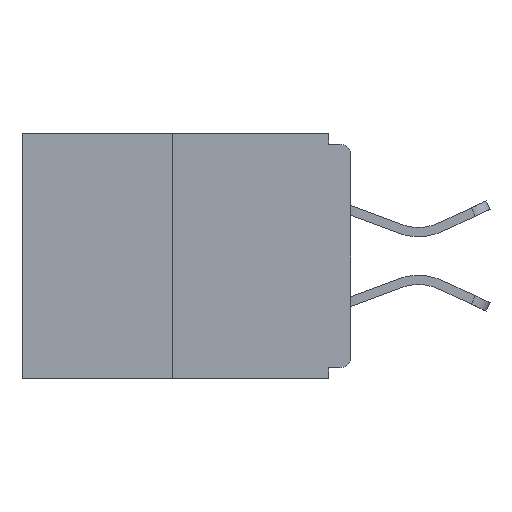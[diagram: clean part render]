
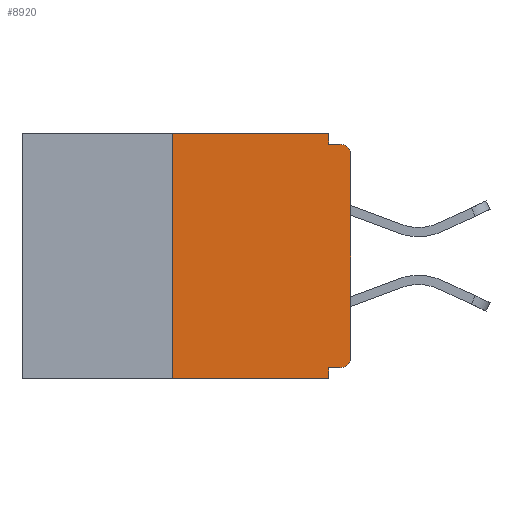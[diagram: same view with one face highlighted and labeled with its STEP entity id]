
A CAD part, left-side view. The second image highlights one B-rep face of the part: STEP entity #8920.
In plain terms, the highlighted planar face has unit normal (-1, 0, 0).
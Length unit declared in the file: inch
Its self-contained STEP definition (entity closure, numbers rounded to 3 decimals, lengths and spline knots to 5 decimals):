
#561 = LINE ( 'NONE', #5467, #5414 ) ;
#595 = VECTOR ( 'NONE', #7251, 39.37008 ) ;
#727 = VERTEX_POINT ( 'NONE', #7992 ) ;
#824 = DIRECTION ( 'NONE',  ( 0., 0., -1. ) ) ;
#912 = VECTOR ( 'NONE', #824, 39.37008 ) ;
#916 = VERTEX_POINT ( 'NONE', #6144 ) ;
#1328 = DIRECTION ( 'NONE',  ( 0., 0., -1. ) ) ;
#1389 = AXIS2_PLACEMENT_3D ( 'NONE', #11991, #3288, #1328 ) ;
#1427 = VECTOR ( 'NONE', #3119, 39.37008 ) ;
#1448 = EDGE_LOOP ( 'NONE', ( #5956, #11105, #6914, #5682, #10189, #10742, #6985, #7976, #5440, #7328 ) ) ;
#1656 = EDGE_CURVE ( 'NONE', #5691, #10394, #11904, .T. ) ;
#1929 = CARTESIAN_POINT ( 'NONE',  ( 0., 0.015, -0.328 ) ) ;
#1949 = PLANE ( 'NONE',  #9711 ) ;
#2046 = FACE_OUTER_BOUND ( 'NONE', #1448, .T. ) ;
#2208 = VERTEX_POINT ( 'NONE', #10287 ) ;
#2291 = CARTESIAN_POINT ( 'NONE',  ( 0., 0., -0.03 ) ) ;
#2743 = CARTESIAN_POINT ( 'NONE',  ( 0., 0.031, 0. ) ) ;
#2788 = DIRECTION ( 'NONE',  ( 0., -1., 0. ) ) ;
#2835 = EDGE_CURVE ( 'NONE', #2208, #5691, #561, .T. ) ;
#3022 = DIRECTION ( 'NONE',  ( 1., 0., 0. ) ) ;
#3119 = DIRECTION ( 'NONE',  ( 0., -1., 0. ) ) ;
#3155 = VERTEX_POINT ( 'NONE', #2291 ) ;
#3254 = CARTESIAN_POINT ( 'NONE',  ( 0., 0.015, -0.015 ) ) ;
#3288 = DIRECTION ( 'NONE',  ( -1., 0., 0. ) ) ;
#3800 = CIRCLE ( 'NONE', #1389, 0.015 ) ;
#3855 = LINE ( 'NONE', #7101, #1427 ) ;
#3993 = DIRECTION ( 'NONE',  ( 0., 0., -1. ) ) ;
#4251 = CARTESIAN_POINT ( 'NONE',  ( 0., 0.031, 0. ) ) ;
#4756 = CARTESIAN_POINT ( 'NONE',  ( 0., 0., -0.328 ) ) ;
#4783 = EDGE_CURVE ( 'NONE', #3155, #12148, #7223, .T. ) ;
#5377 = DIRECTION ( 'NONE',  ( 0., -1., 0. ) ) ;
#5414 = VECTOR ( 'NONE', #11249, 39.37008 ) ;
#5440 = ORIENTED_EDGE ( 'NONE', *, *, #6871, .F. ) ;
#5467 = CARTESIAN_POINT ( 'NONE',  ( 0., 0.25, 0. ) ) ;
#5682 = ORIENTED_EDGE ( 'NONE', *, *, #10095, .F. ) ;
#5691 = VERTEX_POINT ( 'NONE', #10473 ) ;
#5806 = LINE ( 'NONE', #11042, #9380 ) ;
#5827 = EDGE_CURVE ( 'NONE', #10600, #12441, #3800, .T. ) ;
#5956 = ORIENTED_EDGE ( 'NONE', *, *, #1656, .F. ) ;
#6078 = LINE ( 'NONE', #2743, #912 ) ;
#6144 = CARTESIAN_POINT ( 'NONE',  ( 0., 0.031, -0.328 ) ) ;
#6581 = EDGE_CURVE ( 'NONE', #12441, #3155, #10989, .T. ) ;
#6602 = DIRECTION ( 'NONE',  ( 0., 1., 0. ) ) ;
#6702 = CARTESIAN_POINT ( 'NONE',  ( 0., 0.46, 0. ) ) ;
#6709 = CARTESIAN_POINT ( 'NONE',  ( 0., 0., -0.015 ) ) ;
#6871 = EDGE_CURVE ( 'NONE', #12195, #12148, #9323, .T. ) ;
#6914 = ORIENTED_EDGE ( 'NONE', *, *, #11793, .T. ) ;
#6965 = EDGE_CURVE ( 'NONE', #10600, #916, #10816, .T. ) ;
#6985 = ORIENTED_EDGE ( 'NONE', *, *, #6581, .T. ) ;
#7101 = CARTESIAN_POINT ( 'NONE',  ( 0., 0.46, -0.343 ) ) ;
#7223 = CIRCLE ( 'NONE', #8395, 0.015 ) ;
#7251 = DIRECTION ( 'NONE',  ( 0., 0., 1. ) ) ;
#7328 = ORIENTED_EDGE ( 'NONE', *, *, #11694, .F. ) ;
#7502 = CARTESIAN_POINT ( 'NONE',  ( 0., 0.46, 0. ) ) ;
#7670 = DIRECTION ( 'NONE',  ( 0., 0., -1. ) ) ;
#7976 = ORIENTED_EDGE ( 'NONE', *, *, #4783, .T. ) ;
#7992 = CARTESIAN_POINT ( 'NONE',  ( 0., 0.031, -0.343 ) ) ;
#8254 = CARTESIAN_POINT ( 'NONE',  ( 0., 0.031, -0.015 ) ) ;
#8395 = AXIS2_PLACEMENT_3D ( 'NONE', #9520, #12278, #7670 ) ;
#8530 = CARTESIAN_POINT ( 'NONE',  ( 0., 0., -0.313 ) ) ;
#8920 = ADVANCED_FACE ( 'NONE', ( #2046 ), #1949, .F. ) ;
#9323 = LINE ( 'NONE', #6709, #9467 ) ;
#9380 = VECTOR ( 'NONE', #10999, 39.37008 ) ;
#9467 = VECTOR ( 'NONE', #2788, 39.37008 ) ;
#9520 = CARTESIAN_POINT ( 'NONE',  ( 0., 0.015, -0.03 ) ) ;
#9711 = AXIS2_PLACEMENT_3D ( 'NONE', #6702, #3022, #3993 ) ;
#10095 = EDGE_CURVE ( 'NONE', #916, #727, #5806, .T. ) ;
#10189 = ORIENTED_EDGE ( 'NONE', *, *, #6965, .F. ) ;
#10287 = CARTESIAN_POINT ( 'NONE',  ( 0., 0.25, -0.343 ) ) ;
#10394 = VERTEX_POINT ( 'NONE', #4251 ) ;
#10473 = CARTESIAN_POINT ( 'NONE',  ( 0., 0.25, 0. ) ) ;
#10600 = VERTEX_POINT ( 'NONE', #1929 ) ;
#10681 = VECTOR ( 'NONE', #5377, 39.37008 ) ;
#10742 = ORIENTED_EDGE ( 'NONE', *, *, #5827, .T. ) ;
#10816 = LINE ( 'NONE', #4756, #11882 ) ;
#10989 = LINE ( 'NONE', #12057, #595 ) ;
#10999 = DIRECTION ( 'NONE',  ( 0., 0., -1. ) ) ;
#11042 = CARTESIAN_POINT ( 'NONE',  ( 0., 0.031, -0.343 ) ) ;
#11105 = ORIENTED_EDGE ( 'NONE', *, *, #2835, .F. ) ;
#11249 = DIRECTION ( 'NONE',  ( 0., 0., 1. ) ) ;
#11694 = EDGE_CURVE ( 'NONE', #10394, #12195, #6078, .T. ) ;
#11793 = EDGE_CURVE ( 'NONE', #2208, #727, #3855, .T. ) ;
#11882 = VECTOR ( 'NONE', #6602, 39.37008 ) ;
#11904 = LINE ( 'NONE', #7502, #10681 ) ;
#11991 = CARTESIAN_POINT ( 'NONE',  ( 0., 0.015, -0.313 ) ) ;
#12057 = CARTESIAN_POINT ( 'NONE',  ( 0., 0., 0. ) ) ;
#12148 = VERTEX_POINT ( 'NONE', #3254 ) ;
#12195 = VERTEX_POINT ( 'NONE', #8254 ) ;
#12278 = DIRECTION ( 'NONE',  ( -1., 0., 0. ) ) ;
#12441 = VERTEX_POINT ( 'NONE', #8530 ) ;
